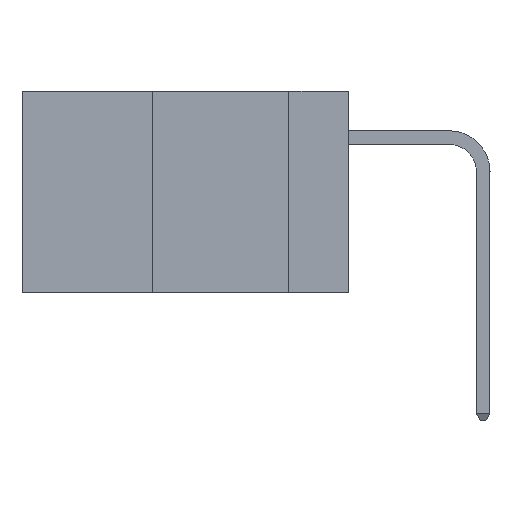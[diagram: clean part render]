
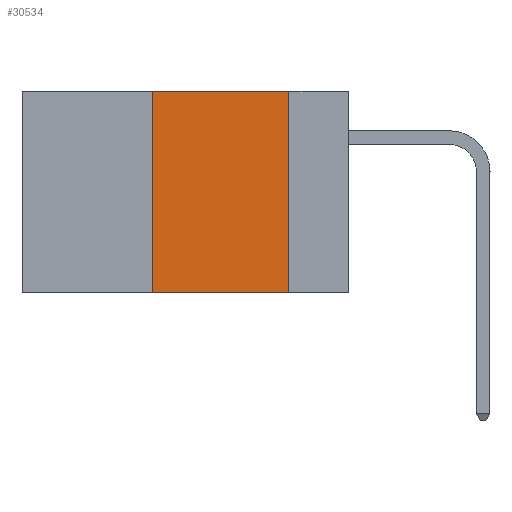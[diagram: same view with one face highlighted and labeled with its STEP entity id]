
A CAD part, left-side view. The second image highlights one B-rep face of the part: STEP entity #30534.
In plain terms, the highlighted planar face has unit normal (-1, 0, 0).
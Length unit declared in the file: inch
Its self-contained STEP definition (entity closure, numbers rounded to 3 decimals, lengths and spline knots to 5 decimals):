
#1038 = EDGE_CURVE ( 'NONE', #30439, #24047, #12971, .T. ) ;
#1781 = VECTOR ( 'NONE', #33171, 39.37008 ) ;
#1963 = CARTESIAN_POINT ( 'NONE',  ( 0., 0.36, 0. ) ) ;
#3226 = DIRECTION ( 'NONE',  ( 0., 0., 1. ) ) ;
#3671 = FACE_OUTER_BOUND ( 'NONE', #26616, .T. ) ;
#5882 = AXIS2_PLACEMENT_3D ( 'NONE', #14993, #34547, #17782 ) ;
#6416 = PLANE ( 'NONE',  #5882 ) ;
#6725 = EDGE_CURVE ( 'NONE', #9339, #25076, #34558, .T. ) ;
#9339 = VERTEX_POINT ( 'NONE', #16769 ) ;
#10498 = CARTESIAN_POINT ( 'NONE',  ( 0., 0.36, 0. ) ) ;
#11346 = DIRECTION ( 'NONE',  ( 0., 0., -1. ) ) ;
#12971 = LINE ( 'NONE', #1963, #26971 ) ;
#13643 = VECTOR ( 'NONE', #34595, 39.37008 ) ;
#14367 = ORIENTED_EDGE ( 'NONE', *, *, #32717, .F. ) ;
#14993 = CARTESIAN_POINT ( 'NONE',  ( 0., 0.6, 0. ) ) ;
#16769 = CARTESIAN_POINT ( 'NONE',  ( 0., 0.11, 0. ) ) ;
#17782 = DIRECTION ( 'NONE',  ( 0., 0., -1. ) ) ;
#21963 = LINE ( 'NONE', #31772, #13643 ) ;
#22513 = CARTESIAN_POINT ( 'NONE',  ( 0., 0.11, 0. ) ) ;
#22587 = ORIENTED_EDGE ( 'NONE', *, *, #35675, .T. ) ;
#24047 = VERTEX_POINT ( 'NONE', #10498 ) ;
#25076 = VERTEX_POINT ( 'NONE', #31930 ) ;
#25087 = LINE ( 'NONE', #30376, #1781 ) ;
#25712 = CARTESIAN_POINT ( 'NONE',  ( 0., 0.36, -0.37 ) ) ;
#26616 = EDGE_LOOP ( 'NONE', ( #27548, #14367, #31687, #22587 ) ) ;
#26971 = VECTOR ( 'NONE', #3226, 39.37008 ) ;
#27081 = VECTOR ( 'NONE', #11346, 39.37008 ) ;
#27548 = ORIENTED_EDGE ( 'NONE', *, *, #6725, .F. ) ;
#30376 = CARTESIAN_POINT ( 'NONE',  ( 0., 0.6, -0.37 ) ) ;
#30439 = VERTEX_POINT ( 'NONE', #25712 ) ;
#30534 = ADVANCED_FACE ( 'NONE', ( #3671 ), #6416, .F. ) ;
#31687 = ORIENTED_EDGE ( 'NONE', *, *, #1038, .F. ) ;
#31772 = CARTESIAN_POINT ( 'NONE',  ( 0., 0.6, 0. ) ) ;
#31930 = CARTESIAN_POINT ( 'NONE',  ( 0., 0.11, -0.37 ) ) ;
#32717 = EDGE_CURVE ( 'NONE', #24047, #9339, #21963, .T. ) ;
#33171 = DIRECTION ( 'NONE',  ( 0., -1., 0. ) ) ;
#34547 = DIRECTION ( 'NONE',  ( 1., 0., 0. ) ) ;
#34558 = LINE ( 'NONE', #22513, #27081 ) ;
#34595 = DIRECTION ( 'NONE',  ( 0., -1., 0. ) ) ;
#35675 = EDGE_CURVE ( 'NONE', #30439, #25076, #25087, .T. ) ;
